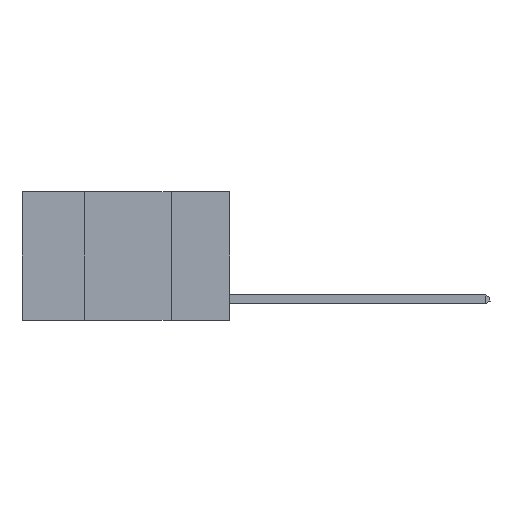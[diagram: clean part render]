
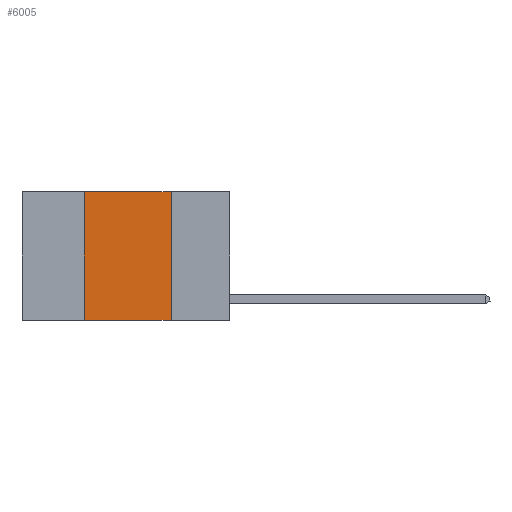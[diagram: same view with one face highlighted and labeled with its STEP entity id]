
A CAD part, left-side view. The second image highlights one B-rep face of the part: STEP entity #6005.
In plain terms, the highlighted planar face has unit normal (-1, 0, 0).
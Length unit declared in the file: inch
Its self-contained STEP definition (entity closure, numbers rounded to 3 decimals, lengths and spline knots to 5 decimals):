
#415 = LINE ( 'NONE', #4247, #6452 ) ;
#891 = VERTEX_POINT ( 'NONE', #3394 ) ;
#1068 = AXIS2_PLACEMENT_3D ( 'NONE', #2518, #9158, #13537 ) ;
#1338 = DIRECTION ( 'NONE',  ( 0., -1., 0. ) ) ;
#1518 = PLANE ( 'NONE',  #1068 ) ;
#1542 = EDGE_CURVE ( 'NONE', #2618, #891, #415, .T. ) ;
#2225 = CARTESIAN_POINT ( 'NONE',  ( 0., 0.17, 0. ) ) ;
#2227 = VECTOR ( 'NONE', #12831, 39.37008 ) ;
#2393 = VERTEX_POINT ( 'NONE', #2225 ) ;
#2441 = CARTESIAN_POINT ( 'NONE',  ( 0., 0.6, -0.37 ) ) ;
#2513 = CARTESIAN_POINT ( 'NONE',  ( 0., 0.17, -0.37 ) ) ;
#2518 = CARTESIAN_POINT ( 'NONE',  ( 0., 0.6, 0. ) ) ;
#2618 = VERTEX_POINT ( 'NONE', #6180 ) ;
#3188 = DIRECTION ( 'NONE',  ( 0., 0., -1. ) ) ;
#3394 = CARTESIAN_POINT ( 'NONE',  ( 0., 0.42, 0. ) ) ;
#3858 = LINE ( 'NONE', #2441, #6283 ) ;
#3947 = VECTOR ( 'NONE', #3188, 39.37008 ) ;
#4247 = CARTESIAN_POINT ( 'NONE',  ( 0., 0.42, 0. ) ) ;
#4302 = EDGE_CURVE ( 'NONE', #2393, #8916, #4442, .T. ) ;
#4442 = LINE ( 'NONE', #6638, #3947 ) ;
#4786 = ORIENTED_EDGE ( 'NONE', *, *, #13533, .T. ) ;
#5861 = ORIENTED_EDGE ( 'NONE', *, *, #10509, .F. ) ;
#6005 = ADVANCED_FACE ( 'NONE', ( #9607 ), #1518, .F. ) ;
#6180 = CARTESIAN_POINT ( 'NONE',  ( 0., 0.42, -0.37 ) ) ;
#6283 = VECTOR ( 'NONE', #1338, 39.37008 ) ;
#6451 = EDGE_LOOP ( 'NONE', ( #7476, #5861, #6790, #4786 ) ) ;
#6452 = VECTOR ( 'NONE', #7428, 39.37008 ) ;
#6638 = CARTESIAN_POINT ( 'NONE',  ( 0., 0.17, 0. ) ) ;
#6790 = ORIENTED_EDGE ( 'NONE', *, *, #1542, .F. ) ;
#7065 = CARTESIAN_POINT ( 'NONE',  ( 0., 0.6, 0. ) ) ;
#7428 = DIRECTION ( 'NONE',  ( 0., 0., 1. ) ) ;
#7476 = ORIENTED_EDGE ( 'NONE', *, *, #4302, .F. ) ;
#8916 = VERTEX_POINT ( 'NONE', #2513 ) ;
#9158 = DIRECTION ( 'NONE',  ( 1., 0., 0. ) ) ;
#9607 = FACE_OUTER_BOUND ( 'NONE', #6451, .T. ) ;
#10509 = EDGE_CURVE ( 'NONE', #891, #2393, #14296, .T. ) ;
#12831 = DIRECTION ( 'NONE',  ( 0., -1., 0. ) ) ;
#13533 = EDGE_CURVE ( 'NONE', #2618, #8916, #3858, .T. ) ;
#13537 = DIRECTION ( 'NONE',  ( 0., 0., -1. ) ) ;
#14296 = LINE ( 'NONE', #7065, #2227 ) ;
